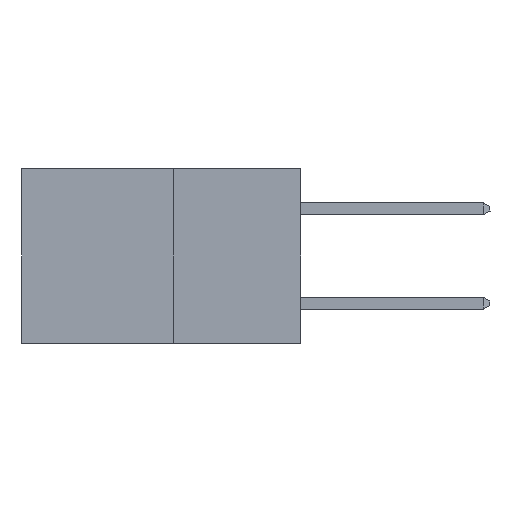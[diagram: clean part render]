
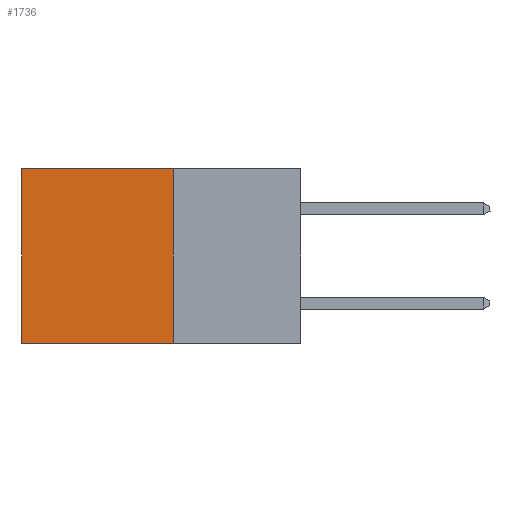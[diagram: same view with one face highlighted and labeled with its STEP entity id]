
A CAD part, left-side view. The second image highlights one B-rep face of the part: STEP entity #1736.
In plain terms, the highlighted planar face has unit normal (-1, 0, 0).
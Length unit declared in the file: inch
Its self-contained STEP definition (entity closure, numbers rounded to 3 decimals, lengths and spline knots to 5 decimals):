
#1327 = LINE ( 'NONE', #8974, #9150 ) ;
#1364 = VERTEX_POINT ( 'NONE', #3627 ) ;
#1736 = ADVANCED_FACE ( 'NONE', ( #5224 ), #7414, .F. ) ;
#2020 = CARTESIAN_POINT ( 'NONE',  ( 0.277, 0.27, -0.37 ) ) ;
#2970 = VECTOR ( 'NONE', #3577, 39.37008 ) ;
#3577 = DIRECTION ( 'NONE',  ( 0., 0., -1. ) ) ;
#3627 = CARTESIAN_POINT ( 'NONE',  ( 0.277, 0.59, 0. ) ) ;
#3691 = DIRECTION ( 'NONE',  ( 0., 0., -1. ) ) ;
#4147 = ORIENTED_EDGE ( 'NONE', *, *, #9541, .F. ) ;
#4313 = VERTEX_POINT ( 'NONE', #12774 ) ;
#4857 = CARTESIAN_POINT ( 'NONE',  ( 0.277, 0.27, -0.37 ) ) ;
#5224 = FACE_OUTER_BOUND ( 'NONE', #19687, .T. ) ;
#6551 = VECTOR ( 'NONE', #13386, 39.37008 ) ;
#6573 = ORIENTED_EDGE ( 'NONE', *, *, #9997, .T. ) ;
#7296 = DIRECTION ( 'NONE',  ( 1., 0., 0. ) ) ;
#7414 = PLANE ( 'NONE',  #8890 ) ;
#8057 = DIRECTION ( 'NONE',  ( 0., 0., -1. ) ) ;
#8890 = AXIS2_PLACEMENT_3D ( 'NONE', #15083, #7296, #8057 ) ;
#8916 = DIRECTION ( 'NONE',  ( 0., 1., 0. ) ) ;
#8974 = CARTESIAN_POINT ( 'NONE',  ( 0.277, 0.27, 0. ) ) ;
#9150 = VECTOR ( 'NONE', #8916, 39.37008 ) ;
#9541 = EDGE_CURVE ( 'NONE', #15495, #4313, #14376, .T. ) ;
#9997 = EDGE_CURVE ( 'NONE', #12965, #1364, #1327, .T. ) ;
#11255 = LINE ( 'NONE', #11452, #14501 ) ;
#11452 = CARTESIAN_POINT ( 'NONE',  ( 0.277, 0.59, -0.37 ) ) ;
#11977 = EDGE_CURVE ( 'NONE', #12965, #15495, #15503, .T. ) ;
#12774 = CARTESIAN_POINT ( 'NONE',  ( 0.277, 0.59, -0.37 ) ) ;
#12965 = VERTEX_POINT ( 'NONE', #15158 ) ;
#13099 = ORIENTED_EDGE ( 'NONE', *, *, #18698, .T. ) ;
#13228 = CARTESIAN_POINT ( 'NONE',  ( 0.277, 0.27, -0.37 ) ) ;
#13386 = DIRECTION ( 'NONE',  ( 0., 1., 0. ) ) ;
#14296 = ORIENTED_EDGE ( 'NONE', *, *, #11977, .F. ) ;
#14376 = LINE ( 'NONE', #13228, #6551 ) ;
#14501 = VECTOR ( 'NONE', #3691, 39.37008 ) ;
#15083 = CARTESIAN_POINT ( 'NONE',  ( 0.277, 0.27, -0.37 ) ) ;
#15158 = CARTESIAN_POINT ( 'NONE',  ( 0.277, 0.27, 0. ) ) ;
#15495 = VERTEX_POINT ( 'NONE', #4857 ) ;
#15503 = LINE ( 'NONE', #2020, #2970 ) ;
#18698 = EDGE_CURVE ( 'NONE', #1364, #4313, #11255, .T. ) ;
#19687 = EDGE_LOOP ( 'NONE', ( #13099, #4147, #14296, #6573 ) ) ;
